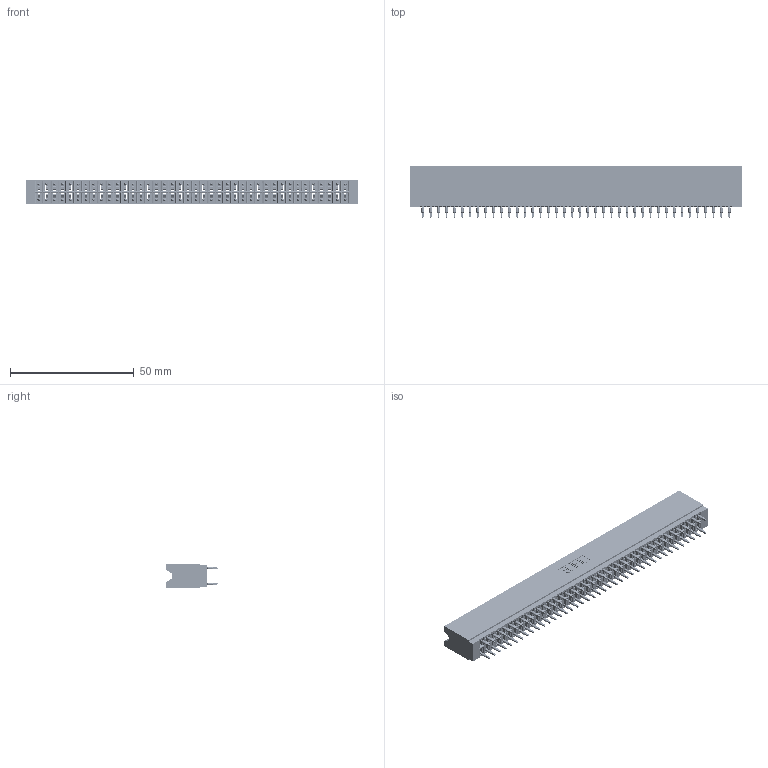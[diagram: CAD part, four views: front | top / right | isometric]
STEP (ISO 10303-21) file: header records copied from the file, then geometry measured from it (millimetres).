
FILE_DESCRIPTION (( 'STEP AP203' ), '1' );
FILE_NAME ('746-080-560-206.STEP', '2026-03-04T16:58:07', ( '' ), ( '' ), 'SwSTEP 2.0', 'SolidWorks 2023', '' );
FILE_SCHEMA (( 'CONFIG_CONTROL_DESIGN' ));
Length unit declared in the file: millimetre
Products named in the file (3): 746-080-560-206; 746 Part_.515 Slot Depth - 06; 746-292-001_560
Assembly tree (81 placements, depth 2):
  746-080-560-206
    746 Part_.515 Slot Depth - 06
    746-292-001_560  x80
Bounding box: 134.24 x 20.82 x 9.91 mm (x, y, z)
Volume: 14656 mm3; surface area: 24816.4 mm2
Topology: 81 solids, 81 shells, 7658 faces, 21305 edges, 13655 vertices
Faces by surface type: plane 3816, cylinder 1762, bspline 1600, torus 480
Entity records: 62216 total; most frequent: CARTESIAN_POINT 12382, ORIENTED_EDGE 10694, DIRECTION 8939, EDGE_CURVE 5347, VECTOR 4755, LINE 4755, VERTEX_POINT 3543, AXIS2_PLACEMENT_3D 2092
